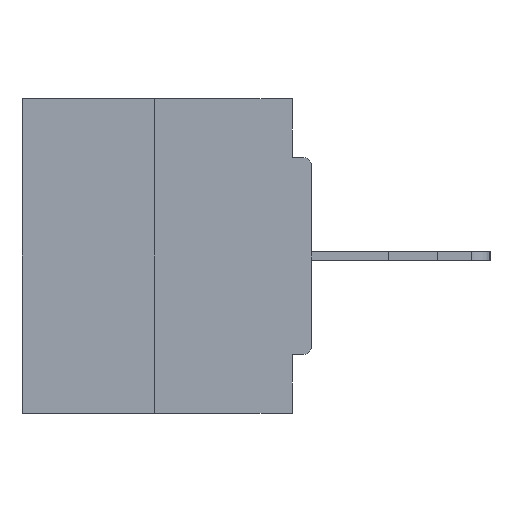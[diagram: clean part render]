
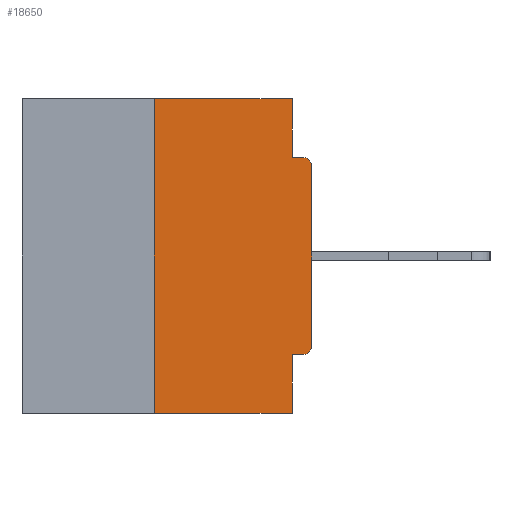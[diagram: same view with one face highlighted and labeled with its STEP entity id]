
A CAD part, left-side view. The second image highlights one B-rep face of the part: STEP entity #18650.
In plain terms, the highlighted planar face has unit normal (-1, 0, 0).
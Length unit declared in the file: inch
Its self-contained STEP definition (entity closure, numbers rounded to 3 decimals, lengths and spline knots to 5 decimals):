
#587 = ORIENTED_EDGE ( 'NONE', *, *, #18375, .T. ) ;
#735 = VERTEX_POINT ( 'NONE', #13862 ) ;
#745 = VERTEX_POINT ( 'NONE', #11988 ) ;
#788 = LINE ( 'NONE', #16571, #27962 ) ;
#964 = AXIS2_PLACEMENT_3D ( 'NONE', #29649, #14449, #32078 ) ;
#1033 = ORIENTED_EDGE ( 'NONE', *, *, #19354, .T. ) ;
#1440 = CARTESIAN_POINT ( 'NONE',  ( 0., 0., 0. ) ) ;
#2387 = DIRECTION ( 'NONE',  ( 0., 0., -1. ) ) ;
#2972 = LINE ( 'NONE', #28822, #23437 ) ;
#3219 = DIRECTION ( 'NONE',  ( 0., 0., 1. ) ) ;
#3479 = PLANE ( 'NONE',  #31032 ) ;
#3649 = CARTESIAN_POINT ( 'NONE',  ( 0., 0.25, -0.5 ) ) ;
#3717 = EDGE_CURVE ( 'NONE', #735, #745, #2972, .T. ) ;
#3948 = LINE ( 'NONE', #28226, #24382 ) ;
#4111 = VERTEX_POINT ( 'NONE', #20099 ) ;
#5744 = EDGE_CURVE ( 'NONE', #21079, #745, #3948, .T. ) ;
#5897 = ORIENTED_EDGE ( 'NONE', *, *, #31050, .F. ) ;
#6008 = CARTESIAN_POINT ( 'NONE',  ( 0., 0.031, 0. ) ) ;
#6062 = DIRECTION ( 'NONE',  ( 0., 0., -1. ) ) ;
#6286 = ORIENTED_EDGE ( 'NONE', *, *, #32280, .F. ) ;
#8487 = EDGE_CURVE ( 'NONE', #23031, #4111, #26964, .T. ) ;
#9044 = DIRECTION ( 'NONE',  ( 0., 1., 0. ) ) ;
#10543 = VERTEX_POINT ( 'NONE', #13612 ) ;
#10788 = VECTOR ( 'NONE', #3219, 39.37008 ) ;
#10818 = VERTEX_POINT ( 'NONE', #22376 ) ;
#10945 = DIRECTION ( 'NONE',  ( 0., -1., 0. ) ) ;
#11167 = LINE ( 'NONE', #26289, #25600 ) ;
#11988 = CARTESIAN_POINT ( 'NONE',  ( 0., 0.031, -0.5 ) ) ;
#13612 = CARTESIAN_POINT ( 'NONE',  ( 0., 0.031, 0. ) ) ;
#13862 = CARTESIAN_POINT ( 'NONE',  ( 0., 0.031, -0.4065 ) ) ;
#13987 = DIRECTION ( 'NONE',  ( 0., -1., 0. ) ) ;
#14449 = DIRECTION ( 'NONE',  ( -1., 0., 0. ) ) ;
#16397 = VERTEX_POINT ( 'NONE', #28469 ) ;
#16571 = CARTESIAN_POINT ( 'NONE',  ( 0., 0.46, 0. ) ) ;
#16606 = EDGE_CURVE ( 'NONE', #27565, #10543, #788, .T. ) ;
#16985 = VERTEX_POINT ( 'NONE', #28222 ) ;
#17018 = ORIENTED_EDGE ( 'NONE', *, *, #8487, .T. ) ;
#17088 = CARTESIAN_POINT ( 'NONE',  ( 0., 0.015, -0.4065 ) ) ;
#17183 = EDGE_CURVE ( 'NONE', #10543, #16397, #29079, .T. ) ;
#17604 = LINE ( 'NONE', #31126, #10788 ) ;
#17725 = DIRECTION ( 'NONE',  ( -1., 0., 0. ) ) ;
#18375 = EDGE_CURVE ( 'NONE', #16985, #10818, #26288, .T. ) ;
#18650 = ADVANCED_FACE ( 'NONE', ( #31644 ), #3479, .F. ) ;
#18961 = EDGE_LOOP ( 'NONE', ( #27356, #24788, #24251, #30958, #6286, #17018, #1033, #587, #5897, #26283 ) ) ;
#19277 = CARTESIAN_POINT ( 'NONE',  ( 0., 0., -0.4065 ) ) ;
#19354 = EDGE_CURVE ( 'NONE', #4111, #16985, #23499, .T. ) ;
#19878 = AXIS2_PLACEMENT_3D ( 'NONE', #32773, #17725, #2387 ) ;
#20099 = CARTESIAN_POINT ( 'NONE',  ( 0., 0., -0.3915 ) ) ;
#20748 = CARTESIAN_POINT ( 'NONE',  ( 0., 0.25, 0. ) ) ;
#21079 = VERTEX_POINT ( 'NONE', #3649 ) ;
#21447 = DIRECTION ( 'NONE',  ( 1., 0., 0. ) ) ;
#22376 = CARTESIAN_POINT ( 'NONE',  ( 0., 0.015, -0.0935 ) ) ;
#22411 = VECTOR ( 'NONE', #31424, 39.37008 ) ;
#22766 = EDGE_CURVE ( 'NONE', #21079, #27565, #17604, .T. ) ;
#23031 = VERTEX_POINT ( 'NONE', #17088 ) ;
#23437 = VECTOR ( 'NONE', #28111, 39.37008 ) ;
#23499 = LINE ( 'NONE', #1440, #29366 ) ;
#24251 = ORIENTED_EDGE ( 'NONE', *, *, #5744, .T. ) ;
#24382 = VECTOR ( 'NONE', #28299, 39.37008 ) ;
#24482 = DIRECTION ( 'NONE',  ( 0., 0., 1. ) ) ;
#24788 = ORIENTED_EDGE ( 'NONE', *, *, #22766, .F. ) ;
#25600 = VECTOR ( 'NONE', #10945, 39.37008 ) ;
#26283 = ORIENTED_EDGE ( 'NONE', *, *, #17183, .F. ) ;
#26288 = CIRCLE ( 'NONE', #19878, 0.015 ) ;
#26289 = CARTESIAN_POINT ( 'NONE',  ( 0., 0., -0.0935 ) ) ;
#26432 = CARTESIAN_POINT ( 'NONE',  ( 0., 0.46, 0. ) ) ;
#26964 = CIRCLE ( 'NONE', #964, 0.015 ) ;
#27056 = LINE ( 'NONE', #19277, #27839 ) ;
#27356 = ORIENTED_EDGE ( 'NONE', *, *, #16606, .F. ) ;
#27565 = VERTEX_POINT ( 'NONE', #20748 ) ;
#27839 = VECTOR ( 'NONE', #9044, 39.37008 ) ;
#27962 = VECTOR ( 'NONE', #13987, 39.37008 ) ;
#28111 = DIRECTION ( 'NONE',  ( 0., 0., -1. ) ) ;
#28222 = CARTESIAN_POINT ( 'NONE',  ( 0., 0., -0.1085 ) ) ;
#28226 = CARTESIAN_POINT ( 'NONE',  ( 0., 0.46, -0.5 ) ) ;
#28299 = DIRECTION ( 'NONE',  ( 0., -1., 0. ) ) ;
#28469 = CARTESIAN_POINT ( 'NONE',  ( 0., 0.031, -0.0935 ) ) ;
#28822 = CARTESIAN_POINT ( 'NONE',  ( 0., 0.031, -0.5 ) ) ;
#29079 = LINE ( 'NONE', #6008, #22411 ) ;
#29366 = VECTOR ( 'NONE', #24482, 39.37008 ) ;
#29649 = CARTESIAN_POINT ( 'NONE',  ( 0., 0.015, -0.3915 ) ) ;
#30958 = ORIENTED_EDGE ( 'NONE', *, *, #3717, .F. ) ;
#31032 = AXIS2_PLACEMENT_3D ( 'NONE', #26432, #21447, #6062 ) ;
#31050 = EDGE_CURVE ( 'NONE', #16397, #10818, #11167, .T. ) ;
#31126 = CARTESIAN_POINT ( 'NONE',  ( 0., 0.25, 0. ) ) ;
#31424 = DIRECTION ( 'NONE',  ( 0., 0., -1. ) ) ;
#31644 = FACE_OUTER_BOUND ( 'NONE', #18961, .T. ) ;
#32078 = DIRECTION ( 'NONE',  ( 0., 0., -1. ) ) ;
#32280 = EDGE_CURVE ( 'NONE', #23031, #735, #27056, .T. ) ;
#32773 = CARTESIAN_POINT ( 'NONE',  ( 0., 0.015, -0.1085 ) ) ;
